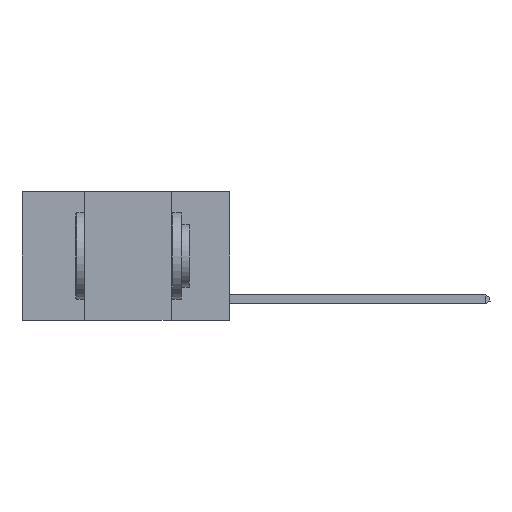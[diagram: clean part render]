
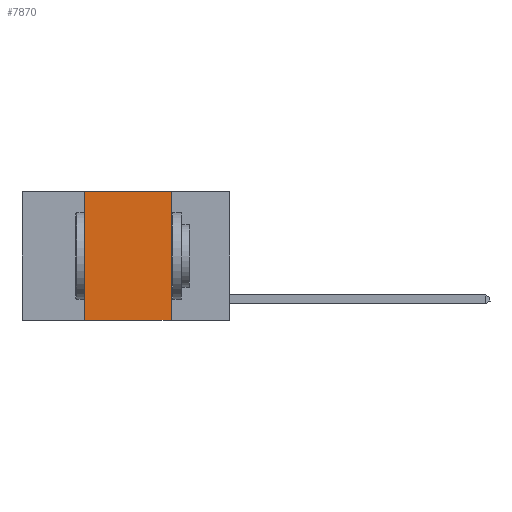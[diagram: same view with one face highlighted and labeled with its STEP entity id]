
A CAD part, left-side view. The second image highlights one B-rep face of the part: STEP entity #7870.
In plain terms, the highlighted planar face has unit normal (-1, 0, 0).
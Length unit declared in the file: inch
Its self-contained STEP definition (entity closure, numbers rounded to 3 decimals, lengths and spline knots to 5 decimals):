
#427 = EDGE_CURVE ( 'NONE', #20263, #7820, #12801, .T. ) ;
#659 = CARTESIAN_POINT ( 'NONE',  ( 0., 0.6, 0. ) ) ;
#943 = EDGE_CURVE ( 'NONE', #7820, #6335, #3690, .T. ) ;
#2055 = LINE ( 'NONE', #14037, #8685 ) ;
#2152 = FACE_OUTER_BOUND ( 'NONE', #13545, .T. ) ;
#3512 = ORIENTED_EDGE ( 'NONE', *, *, #13792, .F. ) ;
#3690 = LINE ( 'NONE', #15570, #12226 ) ;
#4218 = VERTEX_POINT ( 'NONE', #9233 ) ;
#4456 = CARTESIAN_POINT ( 'NONE',  ( 0., 0.17, 0. ) ) ;
#5097 = ORIENTED_EDGE ( 'NONE', *, *, #11002, .T. ) ;
#5307 = VECTOR ( 'NONE', #13763, 39.37008 ) ;
#5611 = PLANE ( 'NONE',  #8552 ) ;
#6335 = VERTEX_POINT ( 'NONE', #21449 ) ;
#6854 = DIRECTION ( 'NONE',  ( 0., 0., 1. ) ) ;
#7609 = ORIENTED_EDGE ( 'NONE', *, *, #427, .F. ) ;
#7808 = VECTOR ( 'NONE', #6854, 39.37008 ) ;
#7820 = VERTEX_POINT ( 'NONE', #4456 ) ;
#7870 = ADVANCED_FACE ( 'NONE', ( #2152 ), #5611, .F. ) ;
#7968 = DIRECTION ( 'NONE',  ( 1., 0., 0. ) ) ;
#8552 = AXIS2_PLACEMENT_3D ( 'NONE', #659, #7968, #13206 ) ;
#8685 = VECTOR ( 'NONE', #8817, 39.37008 ) ;
#8817 = DIRECTION ( 'NONE',  ( 0., -1., 0. ) ) ;
#9233 = CARTESIAN_POINT ( 'NONE',  ( 0., 0.42, -0.37 ) ) ;
#11002 = EDGE_CURVE ( 'NONE', #4218, #6335, #2055, .T. ) ;
#11866 = CARTESIAN_POINT ( 'NONE',  ( 0., 0.42, 0. ) ) ;
#12226 = VECTOR ( 'NONE', #19366, 39.37008 ) ;
#12801 = LINE ( 'NONE', #15650, #5307 ) ;
#13206 = DIRECTION ( 'NONE',  ( 0., 0., -1. ) ) ;
#13545 = EDGE_LOOP ( 'NONE', ( #15932, #7609, #3512, #5097 ) ) ;
#13763 = DIRECTION ( 'NONE',  ( 0., -1., 0. ) ) ;
#13792 = EDGE_CURVE ( 'NONE', #4218, #20263, #20235, .T. ) ;
#14037 = CARTESIAN_POINT ( 'NONE',  ( 0., 0.6, -0.37 ) ) ;
#15570 = CARTESIAN_POINT ( 'NONE',  ( 0., 0.17, 0. ) ) ;
#15650 = CARTESIAN_POINT ( 'NONE',  ( 0., 0.6, 0. ) ) ;
#15932 = ORIENTED_EDGE ( 'NONE', *, *, #943, .F. ) ;
#17094 = CARTESIAN_POINT ( 'NONE',  ( 0., 0.42, 0. ) ) ;
#19366 = DIRECTION ( 'NONE',  ( 0., 0., -1. ) ) ;
#20235 = LINE ( 'NONE', #17094, #7808 ) ;
#20263 = VERTEX_POINT ( 'NONE', #11866 ) ;
#21449 = CARTESIAN_POINT ( 'NONE',  ( 0., 0.17, -0.37 ) ) ;
